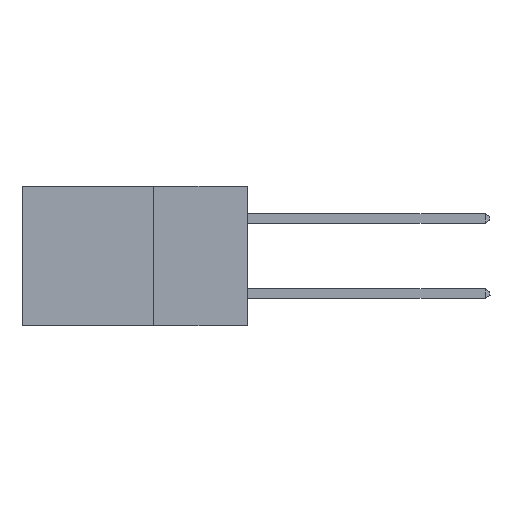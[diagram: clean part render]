
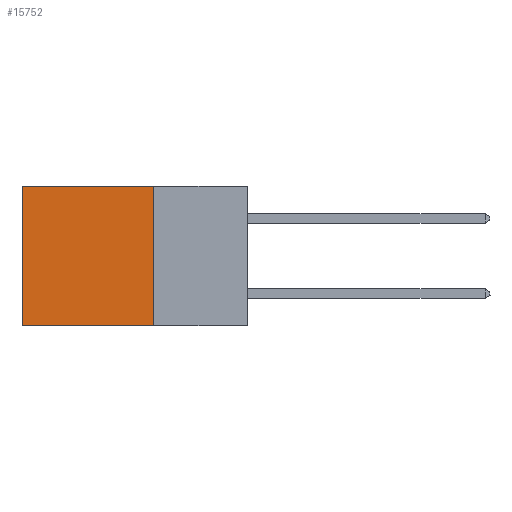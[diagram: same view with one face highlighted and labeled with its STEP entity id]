
A CAD part, left-side view. The second image highlights one B-rep face of the part: STEP entity #15752.
In plain terms, the highlighted planar face has unit normal (-1, 0, 0).
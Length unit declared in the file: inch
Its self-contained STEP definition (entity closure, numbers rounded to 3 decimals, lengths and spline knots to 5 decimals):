
#1297 = DIRECTION ( 'NONE',  ( 0., 1., 0. ) ) ;
#1442 = DIRECTION ( 'NONE',  ( 0., 0., -1. ) ) ;
#1621 = DIRECTION ( 'NONE',  ( 0., 0., -1. ) ) ;
#1695 = LINE ( 'NONE', #20492, #16932 ) ;
#1768 = PLANE ( 'NONE',  #11225 ) ;
#2148 = VERTEX_POINT ( 'NONE', #7590 ) ;
#3841 = VECTOR ( 'NONE', #1621, 39.37008 ) ;
#5617 = VECTOR ( 'NONE', #1297, 39.37008 ) ;
#6538 = CARTESIAN_POINT ( 'NONE',  ( 0.298, 0.25, -0.37 ) ) ;
#6916 = ORIENTED_EDGE ( 'NONE', *, *, #14520, .T. ) ;
#7590 = CARTESIAN_POINT ( 'NONE',  ( 0.298, 0.25, 0. ) ) ;
#7730 = CARTESIAN_POINT ( 'NONE',  ( 0.298, 0.25, 0. ) ) ;
#7849 = DIRECTION ( 'NONE',  ( 0., 0., -1. ) ) ;
#8644 = EDGE_CURVE ( 'NONE', #19976, #25921, #17155, .T. ) ;
#9881 = FACE_OUTER_BOUND ( 'NONE', #14629, .T. ) ;
#10175 = CARTESIAN_POINT ( 'NONE',  ( 0.298, 0.25, 0. ) ) ;
#10747 = EDGE_CURVE ( 'NONE', #2148, #19976, #16074, .T. ) ;
#11225 = AXIS2_PLACEMENT_3D ( 'NONE', #18763, #27043, #7849 ) ;
#13338 = ORIENTED_EDGE ( 'NONE', *, *, #10747, .F. ) ;
#14520 = EDGE_CURVE ( 'NONE', #18519, #25921, #1695, .T. ) ;
#14629 = EDGE_LOOP ( 'NONE', ( #6916, #26121, #13338, #24687 ) ) ;
#15720 = CARTESIAN_POINT ( 'NONE',  ( 0.298, 0.6, -0.37 ) ) ;
#15752 = ADVANCED_FACE ( 'NONE', ( #9881 ), #1768, .F. ) ;
#15797 = CARTESIAN_POINT ( 'NONE',  ( 0.298, 0.25, -0.37 ) ) ;
#15859 = LINE ( 'NONE', #7730, #5617 ) ;
#16074 = LINE ( 'NONE', #10175, #3841 ) ;
#16932 = VECTOR ( 'NONE', #1442, 39.37008 ) ;
#17155 = LINE ( 'NONE', #6538, #25792 ) ;
#18519 = VERTEX_POINT ( 'NONE', #19060 ) ;
#18763 = CARTESIAN_POINT ( 'NONE',  ( 0.298, 0.25, 0. ) ) ;
#19060 = CARTESIAN_POINT ( 'NONE',  ( 0.298, 0.6, 0. ) ) ;
#19976 = VERTEX_POINT ( 'NONE', #15797 ) ;
#20492 = CARTESIAN_POINT ( 'NONE',  ( 0.298, 0.6, 0. ) ) ;
#20758 = EDGE_CURVE ( 'NONE', #2148, #18519, #15859, .T. ) ;
#24687 = ORIENTED_EDGE ( 'NONE', *, *, #20758, .T. ) ;
#25629 = DIRECTION ( 'NONE',  ( 0., 1., 0. ) ) ;
#25792 = VECTOR ( 'NONE', #25629, 39.37008 ) ;
#25921 = VERTEX_POINT ( 'NONE', #15720 ) ;
#26121 = ORIENTED_EDGE ( 'NONE', *, *, #8644, .F. ) ;
#27043 = DIRECTION ( 'NONE',  ( 1., 0., 0. ) ) ;
